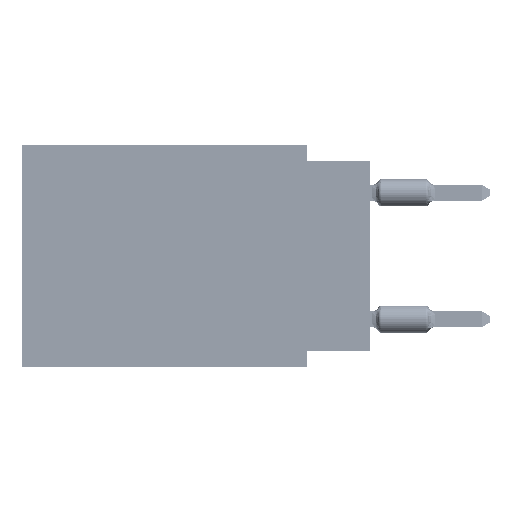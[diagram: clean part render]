
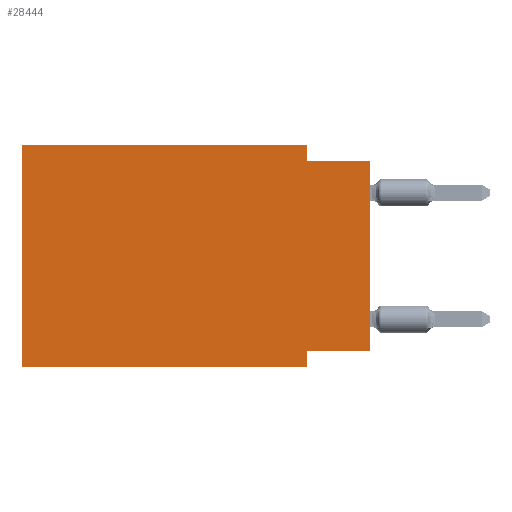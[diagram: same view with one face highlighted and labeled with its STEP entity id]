
A CAD part, left-side view. The second image highlights one B-rep face of the part: STEP entity #28444.
In plain terms, the highlighted planar face has unit normal (-1, 0, 0).
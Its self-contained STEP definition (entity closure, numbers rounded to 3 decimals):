
#3854 = CARTESIAN_POINT ( 'NONE',  ( 0., 2.54, 0. ) ) ;
#5848 = VECTOR ( 'NONE', #109987, 1000. ) ;
#6650 = LINE ( 'NONE', #15882, #49927 ) ;
#11435 = EDGE_CURVE ( 'NONE', #78784, #107694, #82847, .T. ) ;
#13723 = CARTESIAN_POINT ( 'NONE',  ( 0., 0., 0. ) ) ;
#15882 = CARTESIAN_POINT ( 'NONE',  ( 0., 0., -8.255 ) ) ;
#15994 = VECTOR ( 'NONE', #77318, 1000. ) ;
#16210 = LINE ( 'NONE', #70381, #15994 ) ;
#20547 = CARTESIAN_POINT ( 'NONE',  ( 0., 13.97, -8.89 ) ) ;
#20713 = VERTEX_POINT ( 'NONE', #34290 ) ;
#21060 = EDGE_LOOP ( 'NONE', ( #60096, #23731, #105555, #107112, #92675, #81765, #54575, #28041 ) ) ;
#21589 = CARTESIAN_POINT ( 'NONE',  ( 0., 0., -8.255 ) ) ;
#23731 = ORIENTED_EDGE ( 'NONE', *, *, #112515, .F. ) ;
#25952 = LINE ( 'NONE', #61105, #67503 ) ;
#28041 = ORIENTED_EDGE ( 'NONE', *, *, #112236, .F. ) ;
#28444 = ADVANCED_FACE ( 'NONE', ( #64832 ), #45827, .F. ) ;
#31860 = CARTESIAN_POINT ( 'NONE',  ( 0., 13.97, 0. ) ) ;
#32487 = EDGE_CURVE ( 'NONE', #82096, #96504, #74834, .T. ) ;
#32602 = DIRECTION ( 'NONE',  ( 0., 1., 0. ) ) ;
#33493 = VECTOR ( 'NONE', #47932, 1000. ) ;
#34290 = CARTESIAN_POINT ( 'NONE',  ( 0., 2.54, -8.255 ) ) ;
#37612 = EDGE_CURVE ( 'NONE', #20713, #71822, #95407, .T. ) ;
#38053 = EDGE_CURVE ( 'NONE', #88262, #78784, #25952, .T. ) ;
#42939 = CARTESIAN_POINT ( 'NONE',  ( 0., 2.54, -8.89 ) ) ;
#44088 = VECTOR ( 'NONE', #74199, 1000. ) ;
#45124 = CARTESIAN_POINT ( 'NONE',  ( 0., 0., -0.635 ) ) ;
#45827 = PLANE ( 'NONE',  #62569 ) ;
#47932 = DIRECTION ( 'NONE',  ( 0., -1., 0. ) ) ;
#49927 = VECTOR ( 'NONE', #32602, 1000. ) ;
#53382 = CARTESIAN_POINT ( 'NONE',  ( 0., 2.54, -0.635 ) ) ;
#54575 = ORIENTED_EDGE ( 'NONE', *, *, #37612, .F. ) ;
#60096 = ORIENTED_EDGE ( 'NONE', *, *, #32487, .T. ) ;
#60097 = VECTOR ( 'NONE', #78113, 1000. ) ;
#61105 = CARTESIAN_POINT ( 'NONE',  ( 0., 13.97, 0. ) ) ;
#62569 = AXIS2_PLACEMENT_3D ( 'NONE', #81000, #107523, #64253 ) ;
#64253 = DIRECTION ( 'NONE',  ( 0., 0., -1. ) ) ;
#64832 = FACE_OUTER_BOUND ( 'NONE', #21060, .T. ) ;
#67503 = VECTOR ( 'NONE', #96273, 1000. ) ;
#70381 = CARTESIAN_POINT ( 'NONE',  ( 0., 13.97, 0. ) ) ;
#71822 = VERTEX_POINT ( 'NONE', #90978 ) ;
#74199 = DIRECTION ( 'NONE',  ( 0., 0., -1. ) ) ;
#74834 = LINE ( 'NONE', #13723, #5848 ) ;
#75381 = VERTEX_POINT ( 'NONE', #20547 ) ;
#77318 = DIRECTION ( 'NONE',  ( 0., 0., 1. ) ) ;
#78113 = DIRECTION ( 'NONE',  ( 0., 0., -1. ) ) ;
#78784 = VERTEX_POINT ( 'NONE', #83467 ) ;
#80915 = DIRECTION ( 'NONE',  ( 0., -1., 0. ) ) ;
#81000 = CARTESIAN_POINT ( 'NONE',  ( 0., 13.97, 0. ) ) ;
#81765 = ORIENTED_EDGE ( 'NONE', *, *, #90083, .T. ) ;
#82067 = CARTESIAN_POINT ( 'NONE',  ( 0., 13.97, -8.89 ) ) ;
#82096 = VERTEX_POINT ( 'NONE', #21589 ) ;
#82847 = LINE ( 'NONE', #3854, #44088 ) ;
#83467 = CARTESIAN_POINT ( 'NONE',  ( 0., 2.54, 0. ) ) ;
#83663 = LINE ( 'NONE', #100400, #33493 ) ;
#87634 = VECTOR ( 'NONE', #80915, 1000. ) ;
#88262 = VERTEX_POINT ( 'NONE', #31860 ) ;
#90083 = EDGE_CURVE ( 'NONE', #75381, #71822, #98211, .T. ) ;
#90978 = CARTESIAN_POINT ( 'NONE',  ( 0., 2.54, -8.89 ) ) ;
#92675 = ORIENTED_EDGE ( 'NONE', *, *, #105557, .F. ) ;
#95407 = LINE ( 'NONE', #42939, #60097 ) ;
#96273 = DIRECTION ( 'NONE',  ( 0., -1., 0. ) ) ;
#96504 = VERTEX_POINT ( 'NONE', #45124 ) ;
#98211 = LINE ( 'NONE', #82067, #87634 ) ;
#100400 = CARTESIAN_POINT ( 'NONE',  ( 0., 0., -0.635 ) ) ;
#105555 = ORIENTED_EDGE ( 'NONE', *, *, #11435, .F. ) ;
#105557 = EDGE_CURVE ( 'NONE', #75381, #88262, #16210, .T. ) ;
#107112 = ORIENTED_EDGE ( 'NONE', *, *, #38053, .F. ) ;
#107523 = DIRECTION ( 'NONE',  ( 1., 0., 0. ) ) ;
#107694 = VERTEX_POINT ( 'NONE', #53382 ) ;
#109987 = DIRECTION ( 'NONE',  ( 0., 0., 1. ) ) ;
#112236 = EDGE_CURVE ( 'NONE', #82096, #20713, #6650, .T. ) ;
#112515 = EDGE_CURVE ( 'NONE', #107694, #96504, #83663, .T. ) ;
